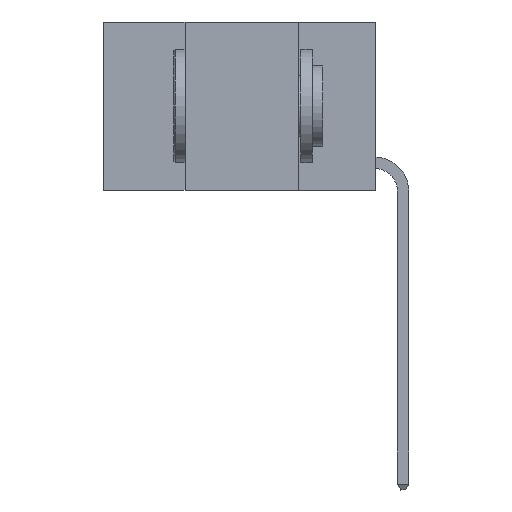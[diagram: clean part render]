
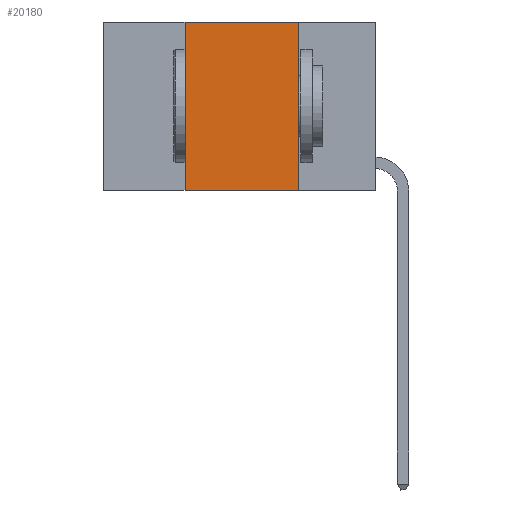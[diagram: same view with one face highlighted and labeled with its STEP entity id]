
A CAD part, left-side view. The second image highlights one B-rep face of the part: STEP entity #20180.
In plain terms, the highlighted planar face has unit normal (-1, 0, 0).
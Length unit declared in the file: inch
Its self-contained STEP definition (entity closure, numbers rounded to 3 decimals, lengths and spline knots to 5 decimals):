
#807 = EDGE_LOOP ( 'NONE', ( #7280, #9671, #900, #26450 ) ) ;
#900 = ORIENTED_EDGE ( 'NONE', *, *, #26955, .F. ) ;
#947 = EDGE_CURVE ( 'NONE', #27083, #6568, #6818, .T. ) ;
#1650 = EDGE_CURVE ( 'NONE', #6568, #1861, #3281, .T. ) ;
#1861 = VERTEX_POINT ( 'NONE', #5138 ) ;
#2048 = DIRECTION ( 'NONE',  ( 0., 0., -1. ) ) ;
#3281 = LINE ( 'NONE', #29917, #15527 ) ;
#4976 = CARTESIAN_POINT ( 'NONE',  ( 0., 0.17, 0. ) ) ;
#5138 = CARTESIAN_POINT ( 'NONE',  ( 0., 0.17, -0.37 ) ) ;
#6248 = PLANE ( 'NONE',  #26227 ) ;
#6413 = CARTESIAN_POINT ( 'NONE',  ( 0., 0.6, 0. ) ) ;
#6449 = CARTESIAN_POINT ( 'NONE',  ( 0., 0.42, 0. ) ) ;
#6568 = VERTEX_POINT ( 'NONE', #4976 ) ;
#6818 = LINE ( 'NONE', #18179, #12905 ) ;
#6831 = VERTEX_POINT ( 'NONE', #23334 ) ;
#7280 = ORIENTED_EDGE ( 'NONE', *, *, #1650, .F. ) ;
#9671 = ORIENTED_EDGE ( 'NONE', *, *, #947, .F. ) ;
#12687 = CARTESIAN_POINT ( 'NONE',  ( 0., 0.42, 0. ) ) ;
#12789 = DIRECTION ( 'NONE',  ( 0., 0., -1. ) ) ;
#12905 = VECTOR ( 'NONE', #13966, 39.37008 ) ;
#13966 = DIRECTION ( 'NONE',  ( 0., -1., 0. ) ) ;
#14546 = EDGE_CURVE ( 'NONE', #6831, #1861, #21633, .T. ) ;
#15527 = VECTOR ( 'NONE', #12789, 39.37008 ) ;
#17096 = VECTOR ( 'NONE', #18818, 39.37008 ) ;
#18160 = VECTOR ( 'NONE', #19868, 39.37008 ) ;
#18179 = CARTESIAN_POINT ( 'NONE',  ( 0., 0.6, 0. ) ) ;
#18818 = DIRECTION ( 'NONE',  ( 0., -1., 0. ) ) ;
#19868 = DIRECTION ( 'NONE',  ( 0., 0., 1. ) ) ;
#20180 = ADVANCED_FACE ( 'NONE', ( #22939 ), #6248, .F. ) ;
#21053 = DIRECTION ( 'NONE',  ( 1., 0., 0. ) ) ;
#21633 = LINE ( 'NONE', #30667, #17096 ) ;
#22939 = FACE_OUTER_BOUND ( 'NONE', #807, .T. ) ;
#23334 = CARTESIAN_POINT ( 'NONE',  ( 0., 0.42, -0.37 ) ) ;
#26227 = AXIS2_PLACEMENT_3D ( 'NONE', #6413, #21053, #2048 ) ;
#26450 = ORIENTED_EDGE ( 'NONE', *, *, #14546, .T. ) ;
#26880 = LINE ( 'NONE', #12687, #18160 ) ;
#26955 = EDGE_CURVE ( 'NONE', #6831, #27083, #26880, .T. ) ;
#27083 = VERTEX_POINT ( 'NONE', #6449 ) ;
#29917 = CARTESIAN_POINT ( 'NONE',  ( 0., 0.17, 0. ) ) ;
#30667 = CARTESIAN_POINT ( 'NONE',  ( 0., 0.6, -0.37 ) ) ;
